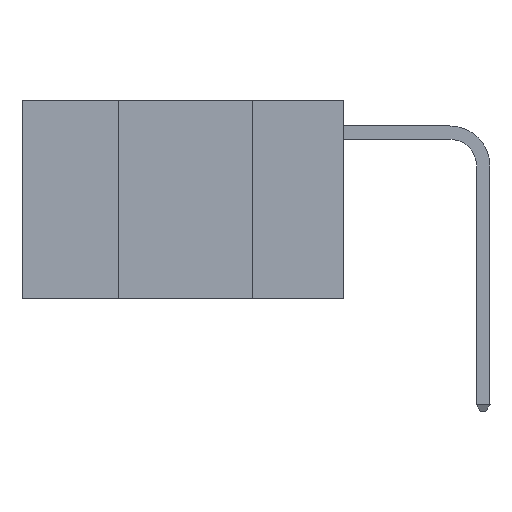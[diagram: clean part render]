
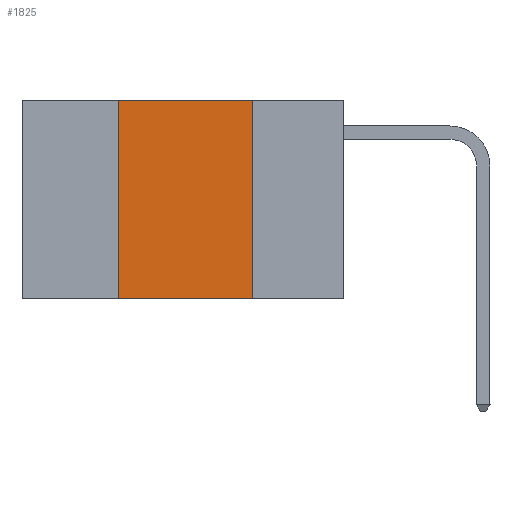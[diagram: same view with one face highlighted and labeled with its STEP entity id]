
A CAD part, left-side view. The second image highlights one B-rep face of the part: STEP entity #1825.
In plain terms, the highlighted planar face has unit normal (-1, 0, 0).
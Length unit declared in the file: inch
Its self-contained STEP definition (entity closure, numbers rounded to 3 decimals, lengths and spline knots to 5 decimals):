
#69 = AXIS2_PLACEMENT_3D ( 'NONE', #10094, #9679, #6852 ) ;
#216 = CARTESIAN_POINT ( 'NONE',  ( 0., 0.17, -0.37 ) ) ;
#727 = CARTESIAN_POINT ( 'NONE',  ( 0., 0.42, 0. ) ) ;
#1492 = VECTOR ( 'NONE', #1560, 39.37008 ) ;
#1560 = DIRECTION ( 'NONE',  ( 0., 0., 1. ) ) ;
#1814 = CARTESIAN_POINT ( 'NONE',  ( 0., 0.42, -0.37 ) ) ;
#1825 = ADVANCED_FACE ( 'NONE', ( #9211 ), #7264, .F. ) ;
#2237 = EDGE_CURVE ( 'NONE', #9696, #6892, #7873, .T. ) ;
#2400 = LINE ( 'NONE', #5658, #4499 ) ;
#2715 = DIRECTION ( 'NONE',  ( 0., -1., 0. ) ) ;
#3189 = CARTESIAN_POINT ( 'NONE',  ( 0., 0.6, 0. ) ) ;
#3298 = DIRECTION ( 'NONE',  ( 0., 0., -1. ) ) ;
#3401 = VECTOR ( 'NONE', #7951, 39.37008 ) ;
#3847 = VERTEX_POINT ( 'NONE', #216 ) ;
#3983 = CARTESIAN_POINT ( 'NONE',  ( 0., 0.42, 0. ) ) ;
#4351 = LINE ( 'NONE', #8290, #8576 ) ;
#4499 = VECTOR ( 'NONE', #3298, 39.37008 ) ;
#4785 = CARTESIAN_POINT ( 'NONE',  ( 0., 0.17, 0. ) ) ;
#5231 = LINE ( 'NONE', #3189, #3401 ) ;
#5658 = CARTESIAN_POINT ( 'NONE',  ( 0., 0.17, 0. ) ) ;
#5807 = ORIENTED_EDGE ( 'NONE', *, *, #2237, .F. ) ;
#6027 = EDGE_LOOP ( 'NONE', ( #8392, #9900, #5807, #6939 ) ) ;
#6372 = EDGE_CURVE ( 'NONE', #9696, #3847, #4351, .T. ) ;
#6852 = DIRECTION ( 'NONE',  ( 0., 0., -1. ) ) ;
#6892 = VERTEX_POINT ( 'NONE', #3983 ) ;
#6939 = ORIENTED_EDGE ( 'NONE', *, *, #6372, .T. ) ;
#6943 = VERTEX_POINT ( 'NONE', #4785 ) ;
#7264 = PLANE ( 'NONE',  #69 ) ;
#7873 = LINE ( 'NONE', #727, #1492 ) ;
#7951 = DIRECTION ( 'NONE',  ( 0., -1., 0. ) ) ;
#8290 = CARTESIAN_POINT ( 'NONE',  ( 0., 0.6, -0.37 ) ) ;
#8392 = ORIENTED_EDGE ( 'NONE', *, *, #10231, .F. ) ;
#8576 = VECTOR ( 'NONE', #2715, 39.37008 ) ;
#9211 = FACE_OUTER_BOUND ( 'NONE', #6027, .T. ) ;
#9679 = DIRECTION ( 'NONE',  ( 1., 0., 0. ) ) ;
#9696 = VERTEX_POINT ( 'NONE', #1814 ) ;
#9900 = ORIENTED_EDGE ( 'NONE', *, *, #10158, .F. ) ;
#10094 = CARTESIAN_POINT ( 'NONE',  ( 0., 0.6, 0. ) ) ;
#10158 = EDGE_CURVE ( 'NONE', #6892, #6943, #5231, .T. ) ;
#10231 = EDGE_CURVE ( 'NONE', #6943, #3847, #2400, .T. ) ;
